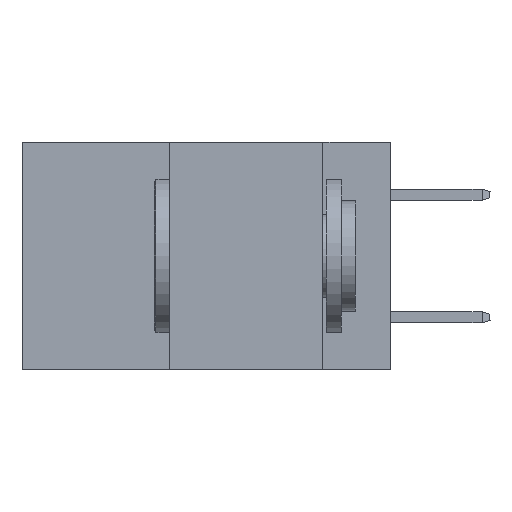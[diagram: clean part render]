
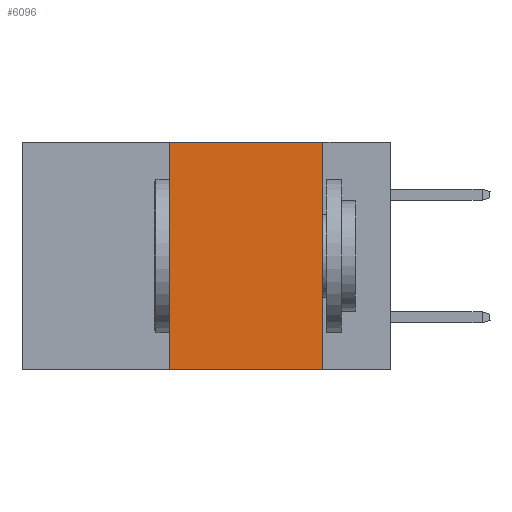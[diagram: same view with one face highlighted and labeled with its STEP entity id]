
A CAD part, left-side view. The second image highlights one B-rep face of the part: STEP entity #6096.
In plain terms, the highlighted planar face has unit normal (-1, 0, 0).
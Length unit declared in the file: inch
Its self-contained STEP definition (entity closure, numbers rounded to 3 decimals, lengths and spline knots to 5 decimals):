
#1192 = EDGE_LOOP ( 'NONE', ( #7247, #16961, #10372, #29975 ) ) ;
#1816 = VERTEX_POINT ( 'NONE', #8155 ) ;
#2176 = CARTESIAN_POINT ( 'NONE',  ( 0., 0.11, 0. ) ) ;
#2252 = VECTOR ( 'NONE', #22387, 39.37008 ) ;
#3110 = CARTESIAN_POINT ( 'NONE',  ( 0., 0.6, -0.37 ) ) ;
#3971 = LINE ( 'NONE', #2176, #32794 ) ;
#5672 = EDGE_CURVE ( 'NONE', #1816, #38263, #6567, .T. ) ;
#6096 = ADVANCED_FACE ( 'NONE', ( #32372 ), #11364, .F. ) ;
#6567 = LINE ( 'NONE', #3110, #37697 ) ;
#6839 = EDGE_CURVE ( 'NONE', #7358, #38263, #3971, .T. ) ;
#7247 = ORIENTED_EDGE ( 'NONE', *, *, #6839, .F. ) ;
#7358 = VERTEX_POINT ( 'NONE', #38777 ) ;
#8155 = CARTESIAN_POINT ( 'NONE',  ( 0., 0.36, -0.37 ) ) ;
#10372 = ORIENTED_EDGE ( 'NONE', *, *, #31074, .F. ) ;
#11364 = PLANE ( 'NONE',  #30335 ) ;
#11663 = LINE ( 'NONE', #14598, #2252 ) ;
#12620 = DIRECTION ( 'NONE',  ( 0., -1., 0. ) ) ;
#14491 = DIRECTION ( 'NONE',  ( 1., 0., 0. ) ) ;
#14598 = CARTESIAN_POINT ( 'NONE',  ( 0., 0.6, 0. ) ) ;
#14722 = DIRECTION ( 'NONE',  ( 0., 0., -1. ) ) ;
#16386 = DIRECTION ( 'NONE',  ( 0., 0., 1. ) ) ;
#16961 = ORIENTED_EDGE ( 'NONE', *, *, #39285, .F. ) ;
#18220 = VECTOR ( 'NONE', #16386, 39.37008 ) ;
#19181 = CARTESIAN_POINT ( 'NONE',  ( 0., 0.11, -0.37 ) ) ;
#22387 = DIRECTION ( 'NONE',  ( 0., -1., 0. ) ) ;
#22621 = VERTEX_POINT ( 'NONE', #38342 ) ;
#26502 = LINE ( 'NONE', #35011, #18220 ) ;
#29975 = ORIENTED_EDGE ( 'NONE', *, *, #5672, .T. ) ;
#30335 = AXIS2_PLACEMENT_3D ( 'NONE', #33126, #14491, #36234 ) ;
#31074 = EDGE_CURVE ( 'NONE', #1816, #22621, #26502, .T. ) ;
#32372 = FACE_OUTER_BOUND ( 'NONE', #1192, .T. ) ;
#32794 = VECTOR ( 'NONE', #14722, 39.37008 ) ;
#33126 = CARTESIAN_POINT ( 'NONE',  ( 0., 0.6, 0. ) ) ;
#35011 = CARTESIAN_POINT ( 'NONE',  ( 0., 0.36, 0. ) ) ;
#36234 = DIRECTION ( 'NONE',  ( 0., 0., -1. ) ) ;
#37697 = VECTOR ( 'NONE', #12620, 39.37008 ) ;
#38263 = VERTEX_POINT ( 'NONE', #19181 ) ;
#38342 = CARTESIAN_POINT ( 'NONE',  ( 0., 0.36, 0. ) ) ;
#38777 = CARTESIAN_POINT ( 'NONE',  ( 0., 0.11, 0. ) ) ;
#39285 = EDGE_CURVE ( 'NONE', #22621, #7358, #11663, .T. ) ;
